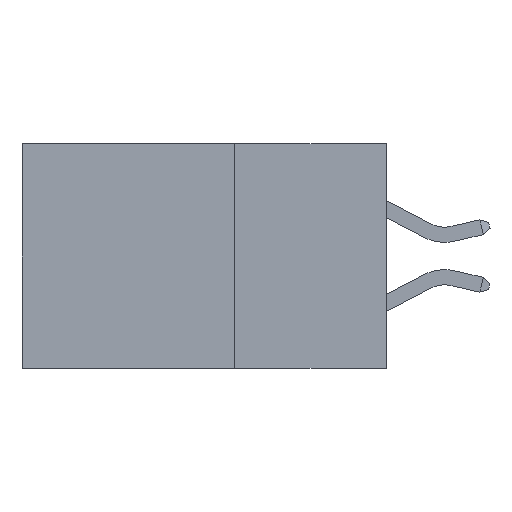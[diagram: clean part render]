
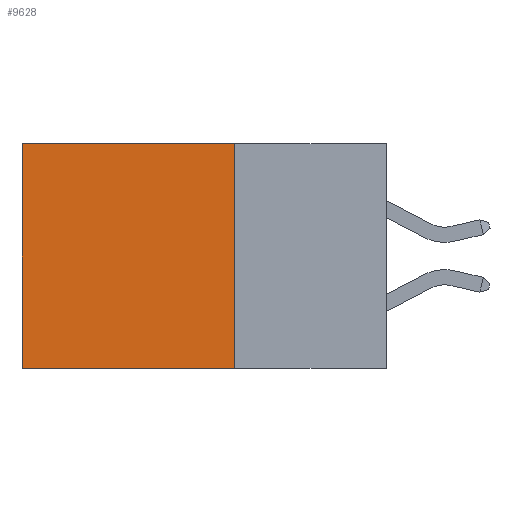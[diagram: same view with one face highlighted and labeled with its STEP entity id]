
A CAD part, left-side view. The second image highlights one B-rep face of the part: STEP entity #9628.
In plain terms, the highlighted planar face has unit normal (-1, 0, 0).
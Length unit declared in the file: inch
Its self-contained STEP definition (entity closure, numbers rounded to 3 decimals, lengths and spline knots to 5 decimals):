
#210 = LINE ( 'NONE', #3466, #12870 ) ;
#977 = CARTESIAN_POINT ( 'NONE',  ( 0.2615, 0.25, -0.37 ) ) ;
#1176 = DIRECTION ( 'NONE',  ( 0., 1., 0. ) ) ;
#1188 = VECTOR ( 'NONE', #1176, 39.37008 ) ;
#1586 = EDGE_CURVE ( 'NONE', #6068, #10397, #210, .T. ) ;
#2503 = ORIENTED_EDGE ( 'NONE', *, *, #10201, .F. ) ;
#2518 = CARTESIAN_POINT ( 'NONE',  ( 0.2615, 0.6, -0.37 ) ) ;
#2618 = CARTESIAN_POINT ( 'NONE',  ( 0.2615, 0.25, 0. ) ) ;
#2620 = DIRECTION ( 'NONE',  ( 0., 1., 0. ) ) ;
#2994 = CARTESIAN_POINT ( 'NONE',  ( 0.2615, 0.25, -0.37 ) ) ;
#3142 = VECTOR ( 'NONE', #12108, 39.37008 ) ;
#3466 = CARTESIAN_POINT ( 'NONE',  ( 0.2615, 0.6, -0.37 ) ) ;
#4167 = DIRECTION ( 'NONE',  ( 0., 0., -1. ) ) ;
#5220 = DIRECTION ( 'NONE',  ( 1., 0., 0. ) ) ;
#5949 = ORIENTED_EDGE ( 'NONE', *, *, #8178, .T. ) ;
#6068 = VERTEX_POINT ( 'NONE', #11754 ) ;
#6098 = FACE_OUTER_BOUND ( 'NONE', #6599, .T. ) ;
#6172 = PLANE ( 'NONE',  #12522 ) ;
#6599 = EDGE_LOOP ( 'NONE', ( #7482, #7159, #2503, #5949 ) ) ;
#7159 = ORIENTED_EDGE ( 'NONE', *, *, #7762, .F. ) ;
#7482 = ORIENTED_EDGE ( 'NONE', *, *, #1586, .T. ) ;
#7637 = LINE ( 'NONE', #977, #3142 ) ;
#7762 = EDGE_CURVE ( 'NONE', #12544, #10397, #11621, .T. ) ;
#8178 = EDGE_CURVE ( 'NONE', #11263, #6068, #12379, .T. ) ;
#8732 = VECTOR ( 'NONE', #2620, 39.37008 ) ;
#9628 = ADVANCED_FACE ( 'NONE', ( #6098 ), #6172, .F. ) ;
#10201 = EDGE_CURVE ( 'NONE', #11263, #12544, #7637, .T. ) ;
#10397 = VERTEX_POINT ( 'NONE', #2518 ) ;
#11263 = VERTEX_POINT ( 'NONE', #2618 ) ;
#11294 = CARTESIAN_POINT ( 'NONE',  ( 0.2615, 0.25, 0. ) ) ;
#11621 = LINE ( 'NONE', #12716, #8732 ) ;
#11754 = CARTESIAN_POINT ( 'NONE',  ( 0.2615, 0.6, 0. ) ) ;
#12077 = CARTESIAN_POINT ( 'NONE',  ( 0.2615, 0.25, -0.37 ) ) ;
#12108 = DIRECTION ( 'NONE',  ( 0., 0., -1. ) ) ;
#12379 = LINE ( 'NONE', #11294, #1188 ) ;
#12522 = AXIS2_PLACEMENT_3D ( 'NONE', #2994, #5220, #4167 ) ;
#12533 = DIRECTION ( 'NONE',  ( 0., 0., -1. ) ) ;
#12544 = VERTEX_POINT ( 'NONE', #12077 ) ;
#12716 = CARTESIAN_POINT ( 'NONE',  ( 0.2615, 0.25, -0.37 ) ) ;
#12870 = VECTOR ( 'NONE', #12533, 39.37008 ) ;
